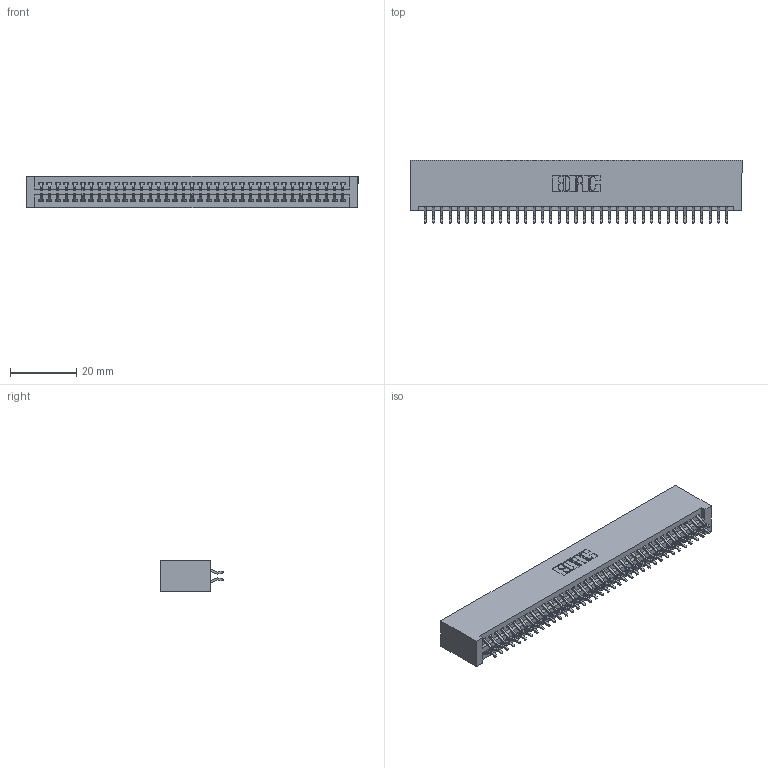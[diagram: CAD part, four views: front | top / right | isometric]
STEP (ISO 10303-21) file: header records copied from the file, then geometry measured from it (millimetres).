
FILE_DESCRIPTION (( 'STEP AP203' ), '1' );
FILE_NAME ('395-074-556-201.STEP', '2018-11-27T19:35:03', ( '' ), ( '' ), 'SwSTEP 2.0', 'SolidWorks 2016', '' );
FILE_SCHEMA (( 'CONFIG_CONTROL_DESIGN' ));
Length unit declared in the file: inch
Products named in the file (3): 345-292-001_556 Tail; 345 Part_No Mounting Lugs; 395-074-556-201
Assembly tree (75 placements, depth 2):
  395-074-556-201
    345 Part_No Mounting Lugs
    345-292-001_556 Tail  x74
Bounding box: 100.58 x 19.24 x 9.4 mm (x, y, z)
Volume: 10337.4 mm3; surface area: 15422.1 mm2
Topology: 75 solids, 75 shells, 4262 faces, 12675 edges, 8350 vertices
Faces by surface type: plane 2814, cylinder 1448
Entity records: 29647 total; most frequent: CARTESIAN_POINT 4988, ORIENTED_EDGE 4910, DIRECTION 4387, EDGE_CURVE 2455, VECTOR 2175, LINE 2175, VERTEX_POINT 1634, AXIS2_PLACEMENT_3D 1106
